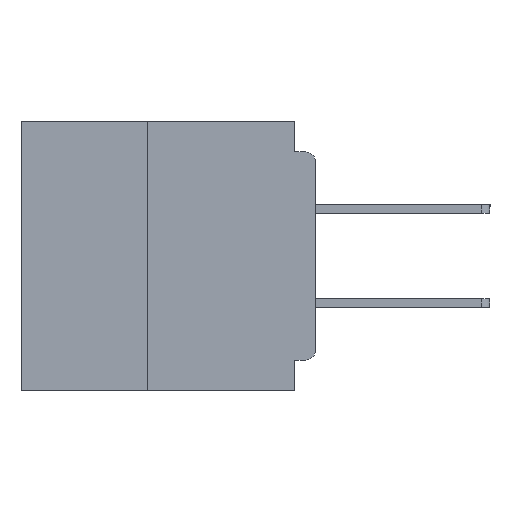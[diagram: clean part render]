
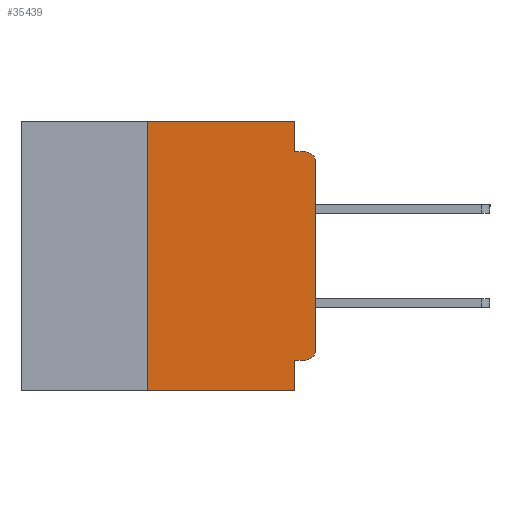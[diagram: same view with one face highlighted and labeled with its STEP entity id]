
A CAD part, left-side view. The second image highlights one B-rep face of the part: STEP entity #35439.
In plain terms, the highlighted planar face has unit normal (-1, 0, 0).
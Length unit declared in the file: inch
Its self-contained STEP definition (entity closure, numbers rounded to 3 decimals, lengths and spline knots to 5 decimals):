
#246 = CARTESIAN_POINT ( 'NONE',  ( 0., 0.031, -0.4 ) ) ;
#728 = LINE ( 'NONE', #9541, #68717 ) ;
#1231 = VERTEX_POINT ( 'NONE', #21853 ) ;
#3321 = VECTOR ( 'NONE', #11819, 39.37008 ) ;
#3949 = ORIENTED_EDGE ( 'NONE', *, *, #17687, .T. ) ;
#5769 = VECTOR ( 'NONE', #57245, 39.37008 ) ;
#6401 = VECTOR ( 'NONE', #40758, 39.37008 ) ;
#8402 = DIRECTION ( 'NONE',  ( -1., 0., 0. ) ) ;
#9066 = CARTESIAN_POINT ( 'NONE',  ( 0., 0.015, -0.045 ) ) ;
#9361 = EDGE_LOOP ( 'NONE', ( #3949, #68763, #65719, #42744, #24300, #11606, #31982, #38355, #42732, #44185 ) ) ;
#9541 = CARTESIAN_POINT ( 'NONE',  ( 0., 0., 0. ) ) ;
#9736 = CIRCLE ( 'NONE', #54905, 0.015 ) ;
#10203 = EDGE_CURVE ( 'NONE', #27555, #34442, #65418, .T. ) ;
#11606 = ORIENTED_EDGE ( 'NONE', *, *, #12266, .F. ) ;
#11711 = LINE ( 'NONE', #31512, #41888 ) ;
#11819 = DIRECTION ( 'NONE',  ( 0., 0., -1. ) ) ;
#12108 = CARTESIAN_POINT ( 'NONE',  ( 0., 0.031, -0.355 ) ) ;
#12266 = EDGE_CURVE ( 'NONE', #27555, #1231, #11711, .T. ) ;
#14021 = EDGE_CURVE ( 'NONE', #29161, #34245, #9736, .T. ) ;
#14342 = CARTESIAN_POINT ( 'NONE',  ( 0., 0., -0.045 ) ) ;
#17687 = EDGE_CURVE ( 'NONE', #34245, #67658, #728, .T. ) ;
#20190 = PLANE ( 'NONE',  #59071 ) ;
#20691 = VECTOR ( 'NONE', #68534, 39.37008 ) ;
#20739 = EDGE_CURVE ( 'NONE', #33151, #64423, #34387, .T. ) ;
#21853 = CARTESIAN_POINT ( 'NONE',  ( 0., 0.25, 0. ) ) ;
#21997 = CARTESIAN_POINT ( 'NONE',  ( 0., 0., -0.06 ) ) ;
#22377 = CARTESIAN_POINT ( 'NONE',  ( 0., 0.031, 0. ) ) ;
#24300 = ORIENTED_EDGE ( 'NONE', *, *, #67323, .F. ) ;
#25592 = DIRECTION ( 'NONE',  ( 0., 0., -1. ) ) ;
#27555 = VERTEX_POINT ( 'NONE', #59035 ) ;
#27916 = CIRCLE ( 'NONE', #44630, 0.015 ) ;
#29161 = VERTEX_POINT ( 'NONE', #48897 ) ;
#29703 = VECTOR ( 'NONE', #65692, 39.37008 ) ;
#30769 = CARTESIAN_POINT ( 'NONE',  ( 0., 0.015, -0.06 ) ) ;
#31512 = CARTESIAN_POINT ( 'NONE',  ( 0., 0.25, -0.4 ) ) ;
#31982 = ORIENTED_EDGE ( 'NONE', *, *, #10203, .T. ) ;
#33151 = VERTEX_POINT ( 'NONE', #66033 ) ;
#33315 = LINE ( 'NONE', #67495, #6401 ) ;
#34245 = VERTEX_POINT ( 'NONE', #41388 ) ;
#34387 = LINE ( 'NONE', #14342, #5769 ) ;
#34442 = VERTEX_POINT ( 'NONE', #246 ) ;
#35418 = EDGE_CURVE ( 'NONE', #67658, #64423, #27916, .T. ) ;
#35439 = ADVANCED_FACE ( 'NONE', ( #40438 ), #20190, .F. ) ;
#36139 = DIRECTION ( 'NONE',  ( 0., 0., -1. ) ) ;
#36920 = VECTOR ( 'NONE', #63892, 39.37008 ) ;
#38355 = ORIENTED_EDGE ( 'NONE', *, *, #59824, .F. ) ;
#40438 = FACE_OUTER_BOUND ( 'NONE', #9361, .T. ) ;
#40501 = CARTESIAN_POINT ( 'NONE',  ( 0., 0.015, -0.34 ) ) ;
#40758 = DIRECTION ( 'NONE',  ( 0., -1., 0. ) ) ;
#41388 = CARTESIAN_POINT ( 'NONE',  ( 0., 0., -0.34 ) ) ;
#41652 = DIRECTION ( 'NONE',  ( 0., 0., 1. ) ) ;
#41888 = VECTOR ( 'NONE', #68915, 39.37008 ) ;
#42732 = ORIENTED_EDGE ( 'NONE', *, *, #45648, .F. ) ;
#42744 = ORIENTED_EDGE ( 'NONE', *, *, #53562, .F. ) ;
#43825 = LINE ( 'NONE', #49519, #29703 ) ;
#44185 = ORIENTED_EDGE ( 'NONE', *, *, #14021, .T. ) ;
#44630 = AXIS2_PLACEMENT_3D ( 'NONE', #30769, #68192, #36139 ) ;
#45648 = EDGE_CURVE ( 'NONE', #29161, #55676, #43825, .T. ) ;
#45869 = DIRECTION ( 'NONE',  ( 0., 0., -1. ) ) ;
#46132 = LINE ( 'NONE', #22377, #3321 ) ;
#48897 = CARTESIAN_POINT ( 'NONE',  ( 0., 0.015, -0.355 ) ) ;
#49519 = CARTESIAN_POINT ( 'NONE',  ( 0., 0., -0.355 ) ) ;
#52054 = CARTESIAN_POINT ( 'NONE',  ( 0., 0.437, 0. ) ) ;
#53562 = EDGE_CURVE ( 'NONE', #54157, #33151, #46132, .T. ) ;
#54157 = VERTEX_POINT ( 'NONE', #68066 ) ;
#54905 = AXIS2_PLACEMENT_3D ( 'NONE', #40501, #8402, #45869 ) ;
#55676 = VERTEX_POINT ( 'NONE', #12108 ) ;
#57245 = DIRECTION ( 'NONE',  ( 0., -1., 0. ) ) ;
#57677 = DIRECTION ( 'NONE',  ( 1., 0., 0. ) ) ;
#58748 = CARTESIAN_POINT ( 'NONE',  ( 0., 0.437, -0.4 ) ) ;
#59035 = CARTESIAN_POINT ( 'NONE',  ( 0., 0.25, -0.4 ) ) ;
#59071 = AXIS2_PLACEMENT_3D ( 'NONE', #52054, #57677, #25592 ) ;
#59824 = EDGE_CURVE ( 'NONE', #55676, #34442, #63446, .T. ) ;
#63169 = CARTESIAN_POINT ( 'NONE',  ( 0., 0.031, -0.4 ) ) ;
#63446 = LINE ( 'NONE', #63169, #20691 ) ;
#63892 = DIRECTION ( 'NONE',  ( 0., -1., 0. ) ) ;
#64423 = VERTEX_POINT ( 'NONE', #9066 ) ;
#65418 = LINE ( 'NONE', #58748, #36920 ) ;
#65692 = DIRECTION ( 'NONE',  ( 0., 1., 0. ) ) ;
#65719 = ORIENTED_EDGE ( 'NONE', *, *, #20739, .F. ) ;
#66033 = CARTESIAN_POINT ( 'NONE',  ( 0., 0.031, -0.045 ) ) ;
#67323 = EDGE_CURVE ( 'NONE', #1231, #54157, #33315, .T. ) ;
#67495 = CARTESIAN_POINT ( 'NONE',  ( 0., 0.437, 0. ) ) ;
#67658 = VERTEX_POINT ( 'NONE', #21997 ) ;
#68066 = CARTESIAN_POINT ( 'NONE',  ( 0., 0.031, 0. ) ) ;
#68192 = DIRECTION ( 'NONE',  ( -1., 0., 0. ) ) ;
#68534 = DIRECTION ( 'NONE',  ( 0., 0., -1. ) ) ;
#68717 = VECTOR ( 'NONE', #41652, 39.37008 ) ;
#68763 = ORIENTED_EDGE ( 'NONE', *, *, #35418, .T. ) ;
#68915 = DIRECTION ( 'NONE',  ( 0., 0., 1. ) ) ;
